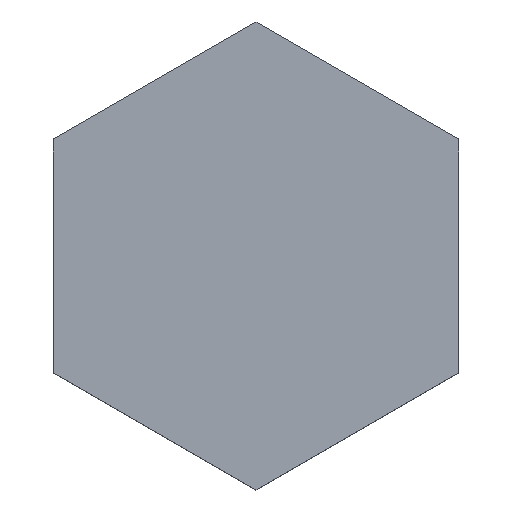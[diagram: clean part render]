
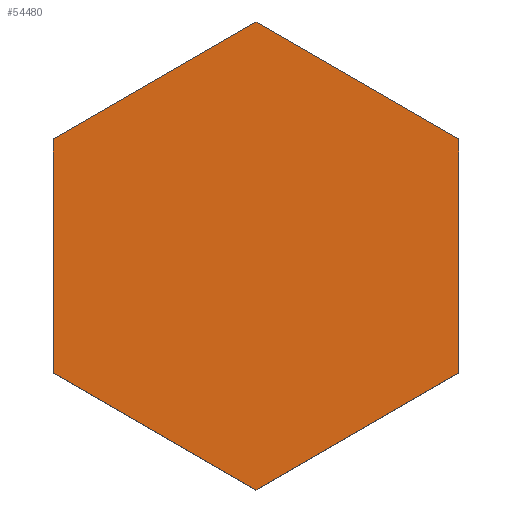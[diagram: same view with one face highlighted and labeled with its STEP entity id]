
A CAD part, top view. The second image highlights one B-rep face of the part: STEP entity #54480.
In plain terms, the highlighted planar face has unit normal (0, 0, 1).
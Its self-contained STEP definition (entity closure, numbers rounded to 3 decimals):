
#54028 = PLANE('',#54029);
#54029 = AXIS2_PLACEMENT_3D('',#54030,#54031,#54032);
#54030 = CARTESIAN_POINT('',(0.,19.05,-151.968));
#54031 = DIRECTION('',(-0.5,0.866,0.));
#54032 = DIRECTION('',(-0.866,-0.5,0.));
#54056 = PLANE('',#54057);
#54057 = AXIS2_PLACEMENT_3D('',#54058,#54059,#54060);
#54058 = CARTESIAN_POINT('',(16.498,9.525,-151.968));
#54059 = DIRECTION('',(0.5,0.866,0.));
#54060 = DIRECTION('',(-0.866,0.5,0.));
#54084 = PLANE('',#54085);
#54085 = AXIS2_PLACEMENT_3D('',#54086,#54087,#54088);
#54086 = CARTESIAN_POINT('',(16.498,-9.525,-151.968));
#54087 = DIRECTION('',(1.,0.,0.));
#54088 = DIRECTION('',(0.,1.,0.));
#54112 = PLANE('',#54113);
#54113 = AXIS2_PLACEMENT_3D('',#54114,#54115,#54116);
#54114 = CARTESIAN_POINT('',(0.,-19.05,-151.968));
#54115 = DIRECTION('',(0.5,-0.866,0.));
#54116 = DIRECTION('',(0.866,0.5,0.));
#54140 = PLANE('',#54141);
#54141 = AXIS2_PLACEMENT_3D('',#54142,#54143,#54144);
#54142 = CARTESIAN_POINT('',(-16.498,-9.525,-151.968));
#54143 = DIRECTION('',(-0.5,-0.866,0.));
#54144 = DIRECTION('',(0.866,-0.5,0.));
#54166 = PLANE('',#54167);
#54167 = AXIS2_PLACEMENT_3D('',#54168,#54169,#54170);
#54168 = CARTESIAN_POINT('',(-16.498,9.525,-151.968));
#54169 = DIRECTION('',(-1.,0.,0.));
#54170 = DIRECTION('',(0.,-1.,0.));
#54186 = VERTEX_POINT('',#54187);
#54187 = CARTESIAN_POINT('',(-16.498,9.525,-151.968));
#54208 = EDGE_CURVE('',#54209,#54186,#54211,.T.);
#54209 = VERTEX_POINT('',#54210);
#54210 = CARTESIAN_POINT('',(0.,19.05,-151.968));
#54211 = SURFACE_CURVE('',#54212,(#54216,#54223),.PCURVE_S1.);
#54212 = LINE('',#54213,#54214);
#54213 = CARTESIAN_POINT('',(0.,19.05,-151.968));
#54214 = VECTOR('',#54215,1.);
#54215 = DIRECTION('',(-0.866,-0.5,0.));
#54216 = PCURVE('',#54028,#54217);
#54217 = DEFINITIONAL_REPRESENTATION('',(#54218),#54222);
#54218 = LINE('',#54219,#54220);
#54219 = CARTESIAN_POINT('',(0.,0.));
#54220 = VECTOR('',#54221,1.);
#54221 = DIRECTION('',(1.,0.));
#54222 = ( GEOMETRIC_REPRESENTATION_CONTEXT(2) 
PARAMETRIC_REPRESENTATION_CONTEXT() REPRESENTATION_CONTEXT('2D SPACE',''
  ) );
#54223 = PCURVE('',#54224,#54229);
#54224 = PLANE('',#54225);
#54225 = AXIS2_PLACEMENT_3D('',#54226,#54227,#54228);
#54226 = CARTESIAN_POINT('',(-7.278,22.416,-151.968));
#54227 = DIRECTION('',(0.,0.,-1.));
#54228 = DIRECTION('',(-1.,0.,0.));
#54229 = DEFINITIONAL_REPRESENTATION('',(#54230),#54234);
#54230 = LINE('',#54231,#54232);
#54231 = CARTESIAN_POINT('',(-7.278,-3.366));
#54232 = VECTOR('',#54233,1.);
#54233 = DIRECTION('',(0.866,-0.5));
#54234 = ( GEOMETRIC_REPRESENTATION_CONTEXT(2) 
PARAMETRIC_REPRESENTATION_CONTEXT() REPRESENTATION_CONTEXT('2D SPACE',''
  ) );
#54262 = EDGE_CURVE('',#54263,#54209,#54265,.T.);
#54263 = VERTEX_POINT('',#54264);
#54264 = CARTESIAN_POINT('',(16.498,9.525,-151.968));
#54265 = SURFACE_CURVE('',#54266,(#54270,#54277),.PCURVE_S1.);
#54266 = LINE('',#54267,#54268);
#54267 = CARTESIAN_POINT('',(16.498,9.525,-151.968));
#54268 = VECTOR('',#54269,1.);
#54269 = DIRECTION('',(-0.866,0.5,0.));
#54270 = PCURVE('',#54056,#54271);
#54271 = DEFINITIONAL_REPRESENTATION('',(#54272),#54276);
#54272 = LINE('',#54273,#54274);
#54273 = CARTESIAN_POINT('',(0.,0.));
#54274 = VECTOR('',#54275,1.);
#54275 = DIRECTION('',(1.,0.));
#54276 = ( GEOMETRIC_REPRESENTATION_CONTEXT(2) 
PARAMETRIC_REPRESENTATION_CONTEXT() REPRESENTATION_CONTEXT('2D SPACE',''
  ) );
#54277 = PCURVE('',#54224,#54278);
#54278 = DEFINITIONAL_REPRESENTATION('',(#54279),#54283);
#54279 = LINE('',#54280,#54281);
#54280 = CARTESIAN_POINT('',(-23.776,-12.891));
#54281 = VECTOR('',#54282,1.);
#54282 = DIRECTION('',(0.866,0.5));
#54283 = ( GEOMETRIC_REPRESENTATION_CONTEXT(2) 
PARAMETRIC_REPRESENTATION_CONTEXT() REPRESENTATION_CONTEXT('2D SPACE',''
  ) );
#54311 = EDGE_CURVE('',#54312,#54263,#54314,.T.);
#54312 = VERTEX_POINT('',#54313);
#54313 = CARTESIAN_POINT('',(16.498,-9.525,-151.968));
#54314 = SURFACE_CURVE('',#54315,(#54319,#54326),.PCURVE_S1.);
#54315 = LINE('',#54316,#54317);
#54316 = CARTESIAN_POINT('',(16.498,-9.525,-151.968));
#54317 = VECTOR('',#54318,1.);
#54318 = DIRECTION('',(0.,1.,0.));
#54319 = PCURVE('',#54084,#54320);
#54320 = DEFINITIONAL_REPRESENTATION('',(#54321),#54325);
#54321 = LINE('',#54322,#54323);
#54322 = CARTESIAN_POINT('',(0.,0.));
#54323 = VECTOR('',#54324,1.);
#54324 = DIRECTION('',(1.,0.));
#54325 = ( GEOMETRIC_REPRESENTATION_CONTEXT(2) 
PARAMETRIC_REPRESENTATION_CONTEXT() REPRESENTATION_CONTEXT('2D SPACE',''
  ) );
#54326 = PCURVE('',#54224,#54327);
#54327 = DEFINITIONAL_REPRESENTATION('',(#54328),#54332);
#54328 = LINE('',#54329,#54330);
#54329 = CARTESIAN_POINT('',(-23.776,-31.941));
#54330 = VECTOR('',#54331,1.);
#54331 = DIRECTION('',(0.,1.));
#54332 = ( GEOMETRIC_REPRESENTATION_CONTEXT(2) 
PARAMETRIC_REPRESENTATION_CONTEXT() REPRESENTATION_CONTEXT('2D SPACE',''
  ) );
#54360 = EDGE_CURVE('',#54361,#54312,#54363,.T.);
#54361 = VERTEX_POINT('',#54362);
#54362 = CARTESIAN_POINT('',(0.,-19.05,-151.968));
#54363 = SURFACE_CURVE('',#54364,(#54368,#54375),.PCURVE_S1.);
#54364 = LINE('',#54365,#54366);
#54365 = CARTESIAN_POINT('',(0.,-19.05,-151.968));
#54366 = VECTOR('',#54367,1.);
#54367 = DIRECTION('',(0.866,0.5,0.));
#54368 = PCURVE('',#54112,#54369);
#54369 = DEFINITIONAL_REPRESENTATION('',(#54370),#54374);
#54370 = LINE('',#54371,#54372);
#54371 = CARTESIAN_POINT('',(0.,0.));
#54372 = VECTOR('',#54373,1.);
#54373 = DIRECTION('',(1.,0.));
#54374 = ( GEOMETRIC_REPRESENTATION_CONTEXT(2) 
PARAMETRIC_REPRESENTATION_CONTEXT() REPRESENTATION_CONTEXT('2D SPACE',''
  ) );
#54375 = PCURVE('',#54224,#54376);
#54376 = DEFINITIONAL_REPRESENTATION('',(#54377),#54381);
#54377 = LINE('',#54378,#54379);
#54378 = CARTESIAN_POINT('',(-7.278,-41.466));
#54379 = VECTOR('',#54380,1.);
#54380 = DIRECTION('',(-0.866,0.5));
#54381 = ( GEOMETRIC_REPRESENTATION_CONTEXT(2) 
PARAMETRIC_REPRESENTATION_CONTEXT() REPRESENTATION_CONTEXT('2D SPACE',''
  ) );
#54409 = EDGE_CURVE('',#54410,#54361,#54412,.T.);
#54410 = VERTEX_POINT('',#54411);
#54411 = CARTESIAN_POINT('',(-16.498,-9.525,-151.968));
#54412 = SURFACE_CURVE('',#54413,(#54417,#54424),.PCURVE_S1.);
#54413 = LINE('',#54414,#54415);
#54414 = CARTESIAN_POINT('',(-16.498,-9.525,-151.968));
#54415 = VECTOR('',#54416,1.);
#54416 = DIRECTION('',(0.866,-0.5,0.));
#54417 = PCURVE('',#54140,#54418);
#54418 = DEFINITIONAL_REPRESENTATION('',(#54419),#54423);
#54419 = LINE('',#54420,#54421);
#54420 = CARTESIAN_POINT('',(0.,0.));
#54421 = VECTOR('',#54422,1.);
#54422 = DIRECTION('',(1.,0.));
#54423 = ( GEOMETRIC_REPRESENTATION_CONTEXT(2) 
PARAMETRIC_REPRESENTATION_CONTEXT() REPRESENTATION_CONTEXT('2D SPACE',''
  ) );
#54424 = PCURVE('',#54224,#54425);
#54425 = DEFINITIONAL_REPRESENTATION('',(#54426),#54430);
#54426 = LINE('',#54427,#54428);
#54427 = CARTESIAN_POINT('',(9.219,-31.941));
#54428 = VECTOR('',#54429,1.);
#54429 = DIRECTION('',(-0.866,-0.5));
#54430 = ( GEOMETRIC_REPRESENTATION_CONTEXT(2) 
PARAMETRIC_REPRESENTATION_CONTEXT() REPRESENTATION_CONTEXT('2D SPACE',''
  ) );
#54458 = EDGE_CURVE('',#54186,#54410,#54459,.T.);
#54459 = SURFACE_CURVE('',#54460,(#54464,#54471),.PCURVE_S1.);
#54460 = LINE('',#54461,#54462);
#54461 = CARTESIAN_POINT('',(-16.498,9.525,-151.968));
#54462 = VECTOR('',#54463,1.);
#54463 = DIRECTION('',(0.,-1.,0.));
#54464 = PCURVE('',#54166,#54465);
#54465 = DEFINITIONAL_REPRESENTATION('',(#54466),#54470);
#54466 = LINE('',#54467,#54468);
#54467 = CARTESIAN_POINT('',(0.,0.));
#54468 = VECTOR('',#54469,1.);
#54469 = DIRECTION('',(1.,0.));
#54470 = ( GEOMETRIC_REPRESENTATION_CONTEXT(2) 
PARAMETRIC_REPRESENTATION_CONTEXT() REPRESENTATION_CONTEXT('2D SPACE',''
  ) );
#54471 = PCURVE('',#54224,#54472);
#54472 = DEFINITIONAL_REPRESENTATION('',(#54473),#54477);
#54473 = LINE('',#54474,#54475);
#54474 = CARTESIAN_POINT('',(9.219,-12.891));
#54475 = VECTOR('',#54476,1.);
#54476 = DIRECTION('',(0.,-1.));
#54477 = ( GEOMETRIC_REPRESENTATION_CONTEXT(2) 
PARAMETRIC_REPRESENTATION_CONTEXT() REPRESENTATION_CONTEXT('2D SPACE',''
  ) );
#54480 = ADVANCED_FACE('',(#54481),#54224,.F.);
#54481 = FACE_BOUND('',#54482,.T.);
#54482 = EDGE_LOOP('',(#54483,#54484,#54485,#54486,#54487,#54488));
#54483 = ORIENTED_EDGE('',*,*,#54409,.T.);
#54484 = ORIENTED_EDGE('',*,*,#54360,.T.);
#54485 = ORIENTED_EDGE('',*,*,#54311,.T.);
#54486 = ORIENTED_EDGE('',*,*,#54262,.T.);
#54487 = ORIENTED_EDGE('',*,*,#54208,.T.);
#54488 = ORIENTED_EDGE('',*,*,#54458,.T.);
